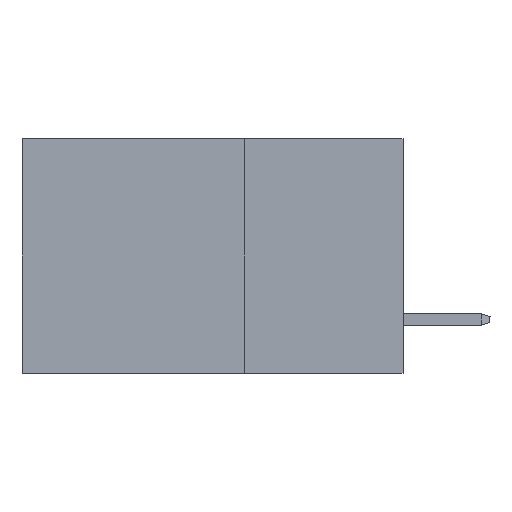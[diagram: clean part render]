
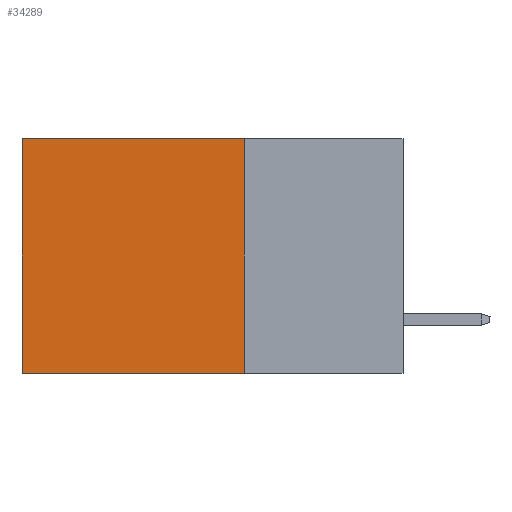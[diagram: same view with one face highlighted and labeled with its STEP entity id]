
A CAD part, left-side view. The second image highlights one B-rep face of the part: STEP entity #34289.
In plain terms, the highlighted planar face has unit normal (-1, 0, 0).
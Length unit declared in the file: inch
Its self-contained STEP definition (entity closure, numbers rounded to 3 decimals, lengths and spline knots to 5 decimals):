
#168 = ORIENTED_EDGE ( 'NONE', *, *, #31873, .F. ) ;
#1129 = DIRECTION ( 'NONE',  ( 0., 0., -1. ) ) ;
#2118 = VERTEX_POINT ( 'NONE', #30567 ) ;
#5117 = LINE ( 'NONE', #20436, #43085 ) ;
#7535 = DIRECTION ( 'NONE',  ( 0., 1., 0. ) ) ;
#7660 = DIRECTION ( 'NONE',  ( 0., 0., -1. ) ) ;
#7762 = DIRECTION ( 'NONE',  ( 1., 0., 0. ) ) ;
#10125 = VERTEX_POINT ( 'NONE', #47588 ) ;
#10811 = VERTEX_POINT ( 'NONE', #12845 ) ;
#11014 = ORIENTED_EDGE ( 'NONE', *, *, #13300, .T. ) ;
#12845 = CARTESIAN_POINT ( 'NONE',  ( 0.2875, 0.6, 0. ) ) ;
#13300 = EDGE_CURVE ( 'NONE', #10811, #2118, #33964, .T. ) ;
#17548 = VECTOR ( 'NONE', #1129, 39.37008 ) ;
#20436 = CARTESIAN_POINT ( 'NONE',  ( 0.2875, 0.25, -0.37 ) ) ;
#20841 = CARTESIAN_POINT ( 'NONE',  ( 0.2875, 0.25, 0. ) ) ;
#21498 = EDGE_LOOP ( 'NONE', ( #11014, #168, #31664, #32786 ) ) ;
#22570 = CARTESIAN_POINT ( 'NONE',  ( 0.2875, 0.25, 0. ) ) ;
#23200 = EDGE_CURVE ( 'NONE', #42502, #10125, #39002, .T. ) ;
#24574 = LINE ( 'NONE', #20841, #31105 ) ;
#27837 = DIRECTION ( 'NONE',  ( 0., 1., 0. ) ) ;
#28212 = CARTESIAN_POINT ( 'NONE',  ( 0.2875, 0.25, 0. ) ) ;
#30567 = CARTESIAN_POINT ( 'NONE',  ( 0.2875, 0.6, -0.37 ) ) ;
#31105 = VECTOR ( 'NONE', #27837, 39.37008 ) ;
#31664 = ORIENTED_EDGE ( 'NONE', *, *, #23200, .F. ) ;
#31873 = EDGE_CURVE ( 'NONE', #10125, #2118, #5117, .T. ) ;
#32786 = ORIENTED_EDGE ( 'NONE', *, *, #48773, .T. ) ;
#33576 = PLANE ( 'NONE',  #44029 ) ;
#33724 = CARTESIAN_POINT ( 'NONE',  ( 0.2875, 0.6, 0. ) ) ;
#33964 = LINE ( 'NONE', #33724, #36965 ) ;
#34289 = ADVANCED_FACE ( 'NONE', ( #34318 ), #33576, .F. ) ;
#34318 = FACE_OUTER_BOUND ( 'NONE', #21498, .T. ) ;
#36965 = VECTOR ( 'NONE', #7660, 39.37008 ) ;
#39002 = LINE ( 'NONE', #28212, #17548 ) ;
#42502 = VERTEX_POINT ( 'NONE', #49167 ) ;
#43085 = VECTOR ( 'NONE', #7535, 39.37008 ) ;
#44029 = AXIS2_PLACEMENT_3D ( 'NONE', #22570, #7762, #45122 ) ;
#45122 = DIRECTION ( 'NONE',  ( 0., 0., -1. ) ) ;
#47588 = CARTESIAN_POINT ( 'NONE',  ( 0.2875, 0.25, -0.37 ) ) ;
#48773 = EDGE_CURVE ( 'NONE', #42502, #10811, #24574, .T. ) ;
#49167 = CARTESIAN_POINT ( 'NONE',  ( 0.2875, 0.25, 0. ) ) ;
